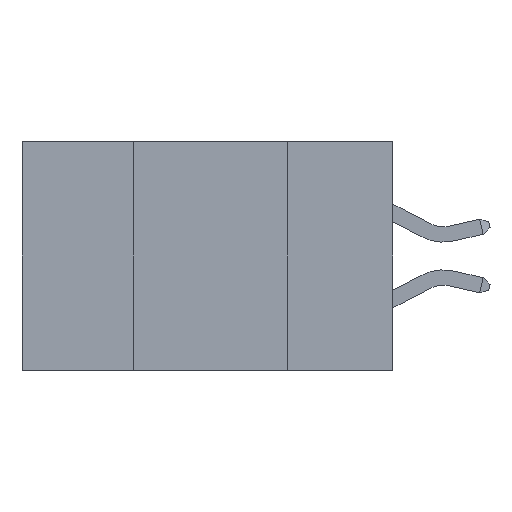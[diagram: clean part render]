
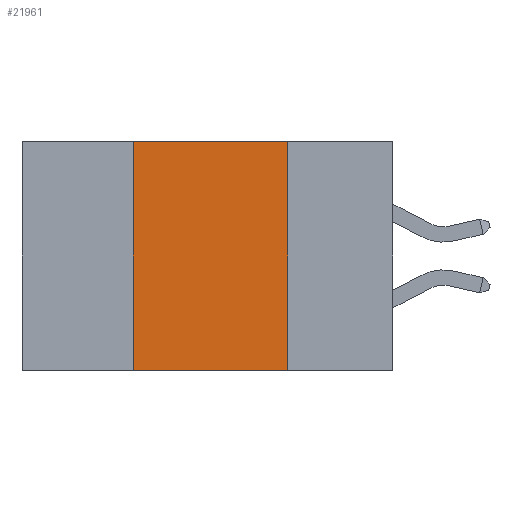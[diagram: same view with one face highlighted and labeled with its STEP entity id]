
A CAD part, left-side view. The second image highlights one B-rep face of the part: STEP entity #21961.
In plain terms, the highlighted planar face has unit normal (-1, 0, 0).
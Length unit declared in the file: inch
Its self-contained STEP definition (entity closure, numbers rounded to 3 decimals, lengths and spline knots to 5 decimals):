
#476 = VERTEX_POINT ( 'NONE', #22787 ) ;
#721 = AXIS2_PLACEMENT_3D ( 'NONE', #5876, #25204, #14569 ) ;
#827 = LINE ( 'NONE', #8493, #23753 ) ;
#2363 = EDGE_CURVE ( 'NONE', #476, #2557, #32569, .T. ) ;
#2557 = VERTEX_POINT ( 'NONE', #10374 ) ;
#4708 = CARTESIAN_POINT ( 'NONE',  ( 0., 0.17, -0.37 ) ) ;
#5876 = CARTESIAN_POINT ( 'NONE',  ( 0., 0.6, 0. ) ) ;
#5927 = EDGE_CURVE ( 'NONE', #25646, #476, #827, .T. ) ;
#8148 = FACE_OUTER_BOUND ( 'NONE', #25218, .T. ) ;
#8240 = DIRECTION ( 'NONE',  ( 0., -1., 0. ) ) ;
#8493 = CARTESIAN_POINT ( 'NONE',  ( 0., 0.42, 0. ) ) ;
#10374 = CARTESIAN_POINT ( 'NONE',  ( 0., 0.17, 0. ) ) ;
#12356 = DIRECTION ( 'NONE',  ( 0., 0., -1. ) ) ;
#12948 = EDGE_CURVE ( 'NONE', #2557, #32483, #28952, .T. ) ;
#14569 = DIRECTION ( 'NONE',  ( 0., 0., -1. ) ) ;
#15104 = DIRECTION ( 'NONE',  ( 0., -1., 0. ) ) ;
#20312 = VECTOR ( 'NONE', #12356, 39.37008 ) ;
#20586 = CARTESIAN_POINT ( 'NONE',  ( 0., 0.17, 0. ) ) ;
#20793 = ORIENTED_EDGE ( 'NONE', *, *, #2363, .F. ) ;
#21191 = EDGE_CURVE ( 'NONE', #25646, #32483, #31128, .T. ) ;
#21961 = ADVANCED_FACE ( 'NONE', ( #8148 ), #33806, .F. ) ;
#22086 = ORIENTED_EDGE ( 'NONE', *, *, #5927, .F. ) ;
#22787 = CARTESIAN_POINT ( 'NONE',  ( 0., 0.42, 0. ) ) ;
#23673 = CARTESIAN_POINT ( 'NONE',  ( 0., 0.6, 0. ) ) ;
#23753 = VECTOR ( 'NONE', #27875, 39.37008 ) ;
#23757 = VECTOR ( 'NONE', #8240, 39.37008 ) ;
#25204 = DIRECTION ( 'NONE',  ( 1., 0., 0. ) ) ;
#25218 = EDGE_LOOP ( 'NONE', ( #35090, #20793, #22086, #27928 ) ) ;
#25646 = VERTEX_POINT ( 'NONE', #33363 ) ;
#26958 = VECTOR ( 'NONE', #15104, 39.37008 ) ;
#27875 = DIRECTION ( 'NONE',  ( 0., 0., 1. ) ) ;
#27928 = ORIENTED_EDGE ( 'NONE', *, *, #21191, .T. ) ;
#28952 = LINE ( 'NONE', #20586, #20312 ) ;
#31128 = LINE ( 'NONE', #32304, #23757 ) ;
#32304 = CARTESIAN_POINT ( 'NONE',  ( 0., 0.6, -0.37 ) ) ;
#32483 = VERTEX_POINT ( 'NONE', #4708 ) ;
#32569 = LINE ( 'NONE', #23673, #26958 ) ;
#33363 = CARTESIAN_POINT ( 'NONE',  ( 0., 0.42, -0.37 ) ) ;
#33806 = PLANE ( 'NONE',  #721 ) ;
#35090 = ORIENTED_EDGE ( 'NONE', *, *, #12948, .F. ) ;
